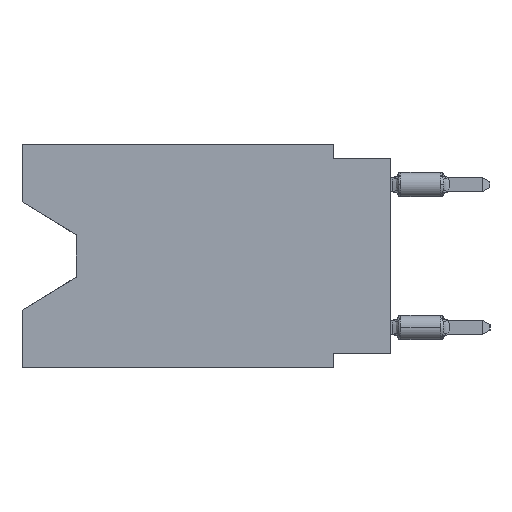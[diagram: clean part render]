
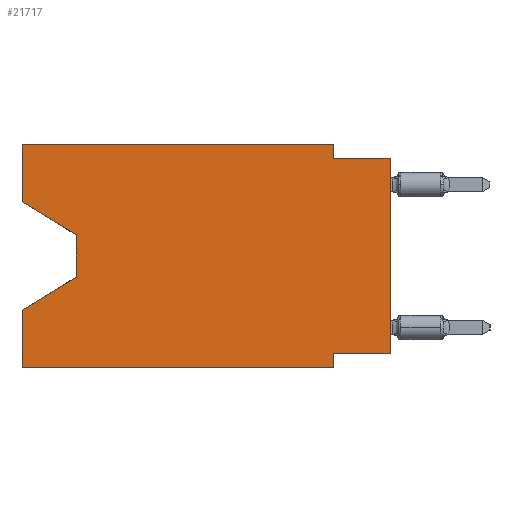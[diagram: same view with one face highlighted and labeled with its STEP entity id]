
A CAD part, left-side view. The second image highlights one B-rep face of the part: STEP entity #21717.
In plain terms, the highlighted planar face has unit normal (-1, 0, 0).
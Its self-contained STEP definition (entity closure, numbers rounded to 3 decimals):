
#26 = CARTESIAN_POINT ( 'NONE',  ( 0., 13.97, -5.893 ) ) ;
#288 = VECTOR ( 'NONE', #29225, 1000. ) ;
#884 = EDGE_LOOP ( 'NONE', ( #32054, #26976, #20367, #18047, #19207, #2014, #6947, #2824, #16665, #24868, #24954, #26650 ) ) ;
#915 = DIRECTION ( 'NONE',  ( 0., 0., 1. ) ) ;
#916 = DIRECTION ( 'NONE',  ( 0., -1., 0. ) ) ;
#1144 = FACE_OUTER_BOUND ( 'NONE', #884, .T. ) ;
#1540 = VERTEX_POINT ( 'NONE', #32287 ) ;
#2014 = ORIENTED_EDGE ( 'NONE', *, *, #3030, .F. ) ;
#2734 = VECTOR ( 'NONE', #14958, 1000. ) ;
#2824 = ORIENTED_EDGE ( 'NONE', *, *, #22632, .T. ) ;
#3030 = EDGE_CURVE ( 'NONE', #22793, #4442, #15552, .T. ) ;
#3671 = DIRECTION ( 'NONE',  ( 0., 0., 1. ) ) ;
#4025 = EDGE_CURVE ( 'NONE', #14466, #5339, #18547, .T. ) ;
#4442 = VERTEX_POINT ( 'NONE', #14368 ) ;
#4533 = EDGE_CURVE ( 'NONE', #5339, #25852, #9088, .T. ) ;
#4691 = VERTEX_POINT ( 'NONE', #32530 ) ;
#4827 = VECTOR ( 'NONE', #18822, 1000. ) ;
#5339 = VERTEX_POINT ( 'NONE', #8120 ) ;
#5652 = VERTEX_POINT ( 'NONE', #9268 ) ;
#6087 = DIRECTION ( 'NONE',  ( 1., 0., 0. ) ) ;
#6881 = LINE ( 'NONE', #31794, #27971 ) ;
#6947 = ORIENTED_EDGE ( 'NONE', *, *, #21012, .F. ) ;
#7702 = VECTOR ( 'NONE', #25868, 1000. ) ;
#7901 = EDGE_CURVE ( 'NONE', #5652, #30786, #14531, .T. ) ;
#8000 = LINE ( 'NONE', #20701, #2734 ) ;
#8120 = CARTESIAN_POINT ( 'NONE',  ( 0., 2.54, 0. ) ) ;
#8133 = VERTEX_POINT ( 'NONE', #26 ) ;
#8884 = CARTESIAN_POINT ( 'NONE',  ( 0., 16.383, 0. ) ) ;
#9088 = LINE ( 'NONE', #29730, #288 ) ;
#9268 = CARTESIAN_POINT ( 'NONE',  ( 0., 16.383, -2.546 ) ) ;
#10080 = EDGE_CURVE ( 'NONE', #30786, #8133, #6881, .T. ) ;
#10979 = CARTESIAN_POINT ( 'NONE',  ( 0., 0., -9.271 ) ) ;
#11491 = DIRECTION ( 'NONE',  ( 0., -1., 0. ) ) ;
#12261 = CARTESIAN_POINT ( 'NONE',  ( 0., 2.54, -9.906 ) ) ;
#12563 = VECTOR ( 'NONE', #3671, 1000. ) ;
#13511 = DIRECTION ( 'NONE',  ( 0., 0., -1. ) ) ;
#13722 = CARTESIAN_POINT ( 'NONE',  ( 0., 16.383, 0. ) ) ;
#14075 = CARTESIAN_POINT ( 'NONE',  ( 0., 16.383, 0. ) ) ;
#14368 = CARTESIAN_POINT ( 'NONE',  ( 0., 2.54, -9.906 ) ) ;
#14443 = EDGE_CURVE ( 'NONE', #1540, #4691, #20831, .T. ) ;
#14466 = VERTEX_POINT ( 'NONE', #13722 ) ;
#14531 = LINE ( 'NONE', #28902, #4827 ) ;
#14958 = DIRECTION ( 'NONE',  ( 0., -1., 0. ) ) ;
#15552 = LINE ( 'NONE', #12261, #21428 ) ;
#16665 = ORIENTED_EDGE ( 'NONE', *, *, #23687, .F. ) ;
#16707 = CARTESIAN_POINT ( 'NONE',  ( 0., 2.54, -0.635 ) ) ;
#16986 = VECTOR ( 'NONE', #17223, 1000. ) ;
#17223 = DIRECTION ( 'NONE',  ( 0., 0., 1. ) ) ;
#18047 = ORIENTED_EDGE ( 'NONE', *, *, #14443, .F. ) ;
#18427 = LINE ( 'NONE', #28830, #7702 ) ;
#18547 = LINE ( 'NONE', #28951, #21270 ) ;
#18822 = DIRECTION ( 'NONE',  ( 0., -0.855, -0.519 ) ) ;
#18970 = CARTESIAN_POINT ( 'NONE',  ( 0., 13.97, -4.013 ) ) ;
#19157 = CARTESIAN_POINT ( 'NONE',  ( 0., 0., -9.271 ) ) ;
#19207 = ORIENTED_EDGE ( 'NONE', *, *, #23423, .T. ) ;
#20367 = ORIENTED_EDGE ( 'NONE', *, *, #22240, .T. ) ;
#20620 = CARTESIAN_POINT ( 'NONE',  ( 0., 16.383, -9.906 ) ) ;
#20701 = CARTESIAN_POINT ( 'NONE',  ( 0., 0., -0.635 ) ) ;
#20831 = LINE ( 'NONE', #30905, #12563 ) ;
#21012 = EDGE_CURVE ( 'NONE', #24369, #22793, #28471, .T. ) ;
#21270 = VECTOR ( 'NONE', #916, 1000. ) ;
#21324 = CARTESIAN_POINT ( 'NONE',  ( 0., 0., -0.635 ) ) ;
#21428 = VECTOR ( 'NONE', #22324, 1000. ) ;
#21662 = VECTOR ( 'NONE', #11491, 1000. ) ;
#21717 = ADVANCED_FACE ( 'NONE', ( #1144 ), #31497, .F. ) ;
#22240 = EDGE_CURVE ( 'NONE', #8133, #4691, #18427, .T. ) ;
#22324 = DIRECTION ( 'NONE',  ( 0., 0., -1. ) ) ;
#22632 = EDGE_CURVE ( 'NONE', #24369, #32119, #23681, .T. ) ;
#22783 = EDGE_CURVE ( 'NONE', #5652, #14466, #24491, .T. ) ;
#22793 = VERTEX_POINT ( 'NONE', #31735 ) ;
#22965 = AXIS2_PLACEMENT_3D ( 'NONE', #8884, #6087, #13511 ) ;
#23348 = CARTESIAN_POINT ( 'NONE',  ( 0., 0., 0. ) ) ;
#23423 = EDGE_CURVE ( 'NONE', #1540, #4442, #23876, .T. ) ;
#23681 = LINE ( 'NONE', #23348, #30694 ) ;
#23687 = EDGE_CURVE ( 'NONE', #25852, #32119, #8000, .T. ) ;
#23876 = LINE ( 'NONE', #20620, #21662 ) ;
#24369 = VERTEX_POINT ( 'NONE', #19157 ) ;
#24491 = LINE ( 'NONE', #14075, #16986 ) ;
#24868 = ORIENTED_EDGE ( 'NONE', *, *, #4533, .F. ) ;
#24954 = ORIENTED_EDGE ( 'NONE', *, *, #4025, .F. ) ;
#25852 = VERTEX_POINT ( 'NONE', #16707 ) ;
#25868 = DIRECTION ( 'NONE',  ( 0., 0.855, -0.519 ) ) ;
#26650 = ORIENTED_EDGE ( 'NONE', *, *, #22783, .F. ) ;
#26976 = ORIENTED_EDGE ( 'NONE', *, *, #10080, .T. ) ;
#27647 = VECTOR ( 'NONE', #30308, 1000. ) ;
#27971 = VECTOR ( 'NONE', #29158, 1000. ) ;
#28471 = LINE ( 'NONE', #10979, #27647 ) ;
#28830 = CARTESIAN_POINT ( 'NONE',  ( 0., 13.97, -5.893 ) ) ;
#28902 = CARTESIAN_POINT ( 'NONE',  ( 0., 16.383, -2.546 ) ) ;
#28951 = CARTESIAN_POINT ( 'NONE',  ( 0., 16.383, 0. ) ) ;
#29158 = DIRECTION ( 'NONE',  ( 0., 0., -1. ) ) ;
#29225 = DIRECTION ( 'NONE',  ( 0., 0., -1. ) ) ;
#29730 = CARTESIAN_POINT ( 'NONE',  ( 0., 2.54, 0. ) ) ;
#30308 = DIRECTION ( 'NONE',  ( 0., 1., 0. ) ) ;
#30694 = VECTOR ( 'NONE', #915, 1000. ) ;
#30786 = VERTEX_POINT ( 'NONE', #18970 ) ;
#30905 = CARTESIAN_POINT ( 'NONE',  ( 0., 16.383, 0. ) ) ;
#31497 = PLANE ( 'NONE',  #22965 ) ;
#31735 = CARTESIAN_POINT ( 'NONE',  ( 0., 2.54, -9.271 ) ) ;
#31794 = CARTESIAN_POINT ( 'NONE',  ( 0., 13.97, -4.013 ) ) ;
#32054 = ORIENTED_EDGE ( 'NONE', *, *, #7901, .T. ) ;
#32119 = VERTEX_POINT ( 'NONE', #21324 ) ;
#32287 = CARTESIAN_POINT ( 'NONE',  ( 0., 16.383, -9.906 ) ) ;
#32530 = CARTESIAN_POINT ( 'NONE',  ( 0., 16.383, -7.36 ) ) ;
